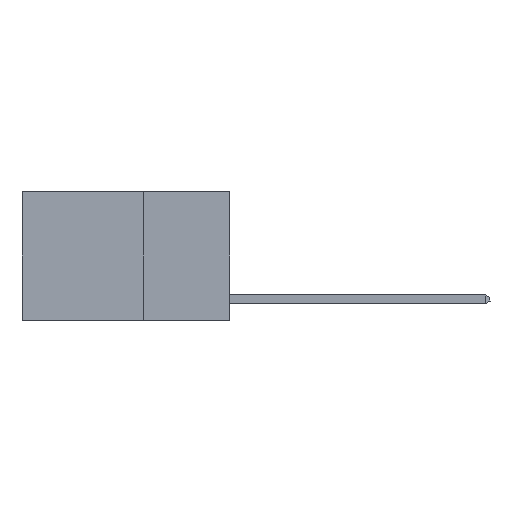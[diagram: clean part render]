
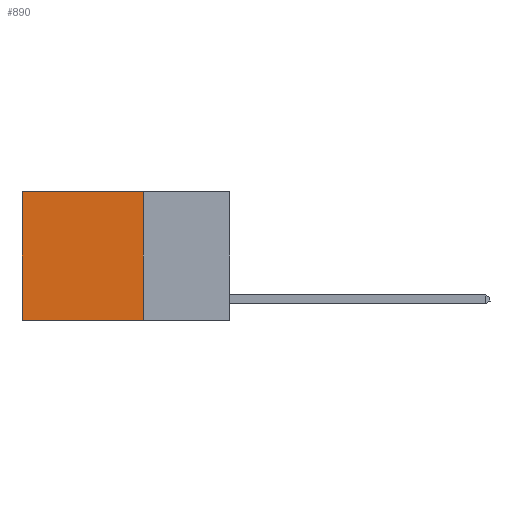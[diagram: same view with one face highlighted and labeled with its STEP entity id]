
A CAD part, left-side view. The second image highlights one B-rep face of the part: STEP entity #890.
In plain terms, the highlighted planar face has unit normal (-1, 0, 0).
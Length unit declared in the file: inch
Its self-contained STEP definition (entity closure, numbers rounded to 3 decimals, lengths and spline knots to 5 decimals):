
#302 = CARTESIAN_POINT ( 'NONE',  ( 0.2625, 0.25, -0.37 ) ) ;
#890 = ADVANCED_FACE ( 'NONE', ( #16678 ), #20975, .F. ) ;
#1123 = LINE ( 'NONE', #302, #15978 ) ;
#1403 = CARTESIAN_POINT ( 'NONE',  ( 0.2625, 0.25, 0. ) ) ;
#2057 = VERTEX_POINT ( 'NONE', #4389 ) ;
#2672 = VERTEX_POINT ( 'NONE', #13190 ) ;
#4389 = CARTESIAN_POINT ( 'NONE',  ( 0.2625, 0.25, -0.37 ) ) ;
#5255 = VECTOR ( 'NONE', #20217, 39.37008 ) ;
#5840 = LINE ( 'NONE', #5953, #5255 ) ;
#5953 = CARTESIAN_POINT ( 'NONE',  ( 0.2625, 0.25, 0. ) ) ;
#6791 = CARTESIAN_POINT ( 'NONE',  ( 0.2625, 0.25, 0. ) ) ;
#7616 = EDGE_CURVE ( 'NONE', #17080, #2057, #8213, .T. ) ;
#7707 = EDGE_LOOP ( 'NONE', ( #13165, #22867, #19156, #19710 ) ) ;
#8006 = VECTOR ( 'NONE', #9498, 39.37008 ) ;
#8204 = CARTESIAN_POINT ( 'NONE',  ( 0.2625, 0.25, 0. ) ) ;
#8213 = LINE ( 'NONE', #8204, #16025 ) ;
#8535 = EDGE_CURVE ( 'NONE', #2057, #16766, #1123, .T. ) ;
#8575 = DIRECTION ( 'NONE',  ( 0., 0., -1. ) ) ;
#9498 = DIRECTION ( 'NONE',  ( 0., 0., -1. ) ) ;
#10747 = EDGE_CURVE ( 'NONE', #17080, #2672, #5840, .T. ) ;
#13121 = CARTESIAN_POINT ( 'NONE',  ( 0.2625, 0.6, -0.37 ) ) ;
#13165 = ORIENTED_EDGE ( 'NONE', *, *, #23058, .T. ) ;
#13190 = CARTESIAN_POINT ( 'NONE',  ( 0.2625, 0.6, 0. ) ) ;
#13513 = DIRECTION ( 'NONE',  ( 0., 0., -1. ) ) ;
#13999 = AXIS2_PLACEMENT_3D ( 'NONE', #6791, #19268, #8575 ) ;
#15978 = VECTOR ( 'NONE', #20038, 39.37008 ) ;
#16025 = VECTOR ( 'NONE', #13513, 39.37008 ) ;
#16656 = CARTESIAN_POINT ( 'NONE',  ( 0.2625, 0.6, 0. ) ) ;
#16678 = FACE_OUTER_BOUND ( 'NONE', #7707, .T. ) ;
#16766 = VERTEX_POINT ( 'NONE', #13121 ) ;
#16944 = LINE ( 'NONE', #16656, #8006 ) ;
#17080 = VERTEX_POINT ( 'NONE', #1403 ) ;
#19156 = ORIENTED_EDGE ( 'NONE', *, *, #7616, .F. ) ;
#19268 = DIRECTION ( 'NONE',  ( 1., 0., 0. ) ) ;
#19710 = ORIENTED_EDGE ( 'NONE', *, *, #10747, .T. ) ;
#20038 = DIRECTION ( 'NONE',  ( 0., 1., 0. ) ) ;
#20217 = DIRECTION ( 'NONE',  ( 0., 1., 0. ) ) ;
#20975 = PLANE ( 'NONE',  #13999 ) ;
#22867 = ORIENTED_EDGE ( 'NONE', *, *, #8535, .F. ) ;
#23058 = EDGE_CURVE ( 'NONE', #2672, #16766, #16944, .T. ) ;
